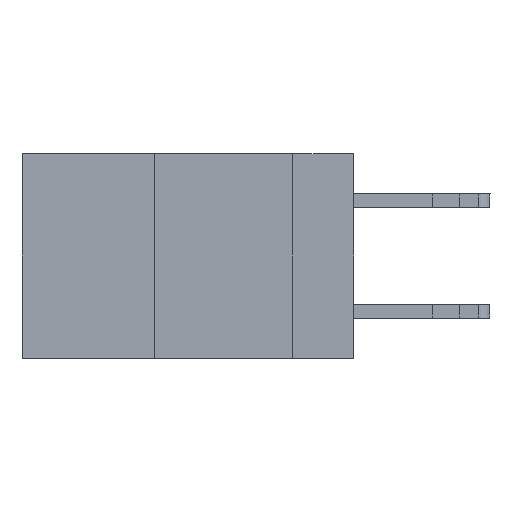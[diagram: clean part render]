
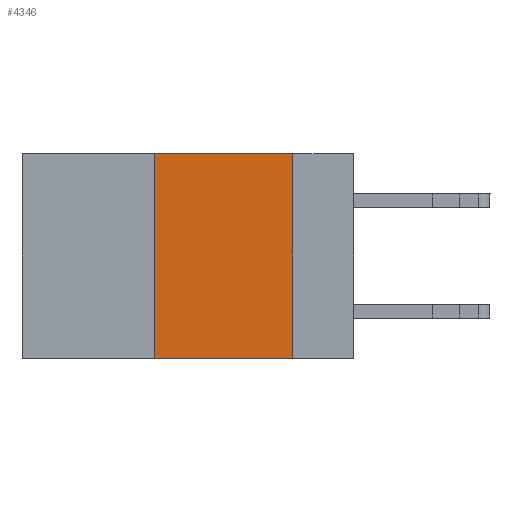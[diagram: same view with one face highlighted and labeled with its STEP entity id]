
A CAD part, left-side view. The second image highlights one B-rep face of the part: STEP entity #4346.
In plain terms, the highlighted planar face has unit normal (-1, 0, 0).
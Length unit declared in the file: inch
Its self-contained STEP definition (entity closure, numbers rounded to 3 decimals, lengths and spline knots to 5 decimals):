
#1619 = VECTOR ( 'NONE', #9592, 39.37008 ) ;
#1938 = VERTEX_POINT ( 'NONE', #3108 ) ;
#2101 = CARTESIAN_POINT ( 'NONE',  ( 0., 0.36, 0. ) ) ;
#2422 = EDGE_CURVE ( 'NONE', #11448, #7695, #15321, .T. ) ;
#2758 = CARTESIAN_POINT ( 'NONE',  ( 0., 0.11, -0.37 ) ) ;
#3108 = CARTESIAN_POINT ( 'NONE',  ( 0., 0.36, 0. ) ) ;
#4346 = ADVANCED_FACE ( 'NONE', ( #6828 ), #11741, .F. ) ;
#4435 = DIRECTION ( 'NONE',  ( 0., 0., -1. ) ) ;
#4913 = EDGE_CURVE ( 'NONE', #14951, #7695, #10792, .T. ) ;
#5261 = CARTESIAN_POINT ( 'NONE',  ( 0., 0.6, 0. ) ) ;
#5479 = EDGE_LOOP ( 'NONE', ( #7850, #7207, #13230, #13426 ) ) ;
#5728 = AXIS2_PLACEMENT_3D ( 'NONE', #7789, #10528, #4435 ) ;
#6042 = DIRECTION ( 'NONE',  ( 0., 0., 1. ) ) ;
#6828 = FACE_OUTER_BOUND ( 'NONE', #5479, .T. ) ;
#6985 = CARTESIAN_POINT ( 'NONE',  ( 0., 0.11, 0. ) ) ;
#7207 = ORIENTED_EDGE ( 'NONE', *, *, #12472, .F. ) ;
#7695 = VERTEX_POINT ( 'NONE', #2758 ) ;
#7789 = CARTESIAN_POINT ( 'NONE',  ( 0., 0.6, 0. ) ) ;
#7850 = ORIENTED_EDGE ( 'NONE', *, *, #4913, .F. ) ;
#8450 = VECTOR ( 'NONE', #6042, 39.37008 ) ;
#9592 = DIRECTION ( 'NONE',  ( 0., 0., -1. ) ) ;
#9771 = VECTOR ( 'NONE', #15555, 39.37008 ) ;
#10160 = DIRECTION ( 'NONE',  ( 0., -1., 0. ) ) ;
#10528 = DIRECTION ( 'NONE',  ( 1., 0., 0. ) ) ;
#10792 = LINE ( 'NONE', #14508, #1619 ) ;
#10986 = CARTESIAN_POINT ( 'NONE',  ( 0., 0.36, -0.37 ) ) ;
#11448 = VERTEX_POINT ( 'NONE', #10986 ) ;
#11741 = PLANE ( 'NONE',  #5728 ) ;
#12237 = VECTOR ( 'NONE', #10160, 39.37008 ) ;
#12472 = EDGE_CURVE ( 'NONE', #1938, #14951, #14918, .T. ) ;
#13230 = ORIENTED_EDGE ( 'NONE', *, *, #14507, .F. ) ;
#13426 = ORIENTED_EDGE ( 'NONE', *, *, #2422, .T. ) ;
#14261 = CARTESIAN_POINT ( 'NONE',  ( 0., 0.6, -0.37 ) ) ;
#14488 = LINE ( 'NONE', #2101, #8450 ) ;
#14507 = EDGE_CURVE ( 'NONE', #11448, #1938, #14488, .T. ) ;
#14508 = CARTESIAN_POINT ( 'NONE',  ( 0., 0.11, 0. ) ) ;
#14918 = LINE ( 'NONE', #5261, #12237 ) ;
#14951 = VERTEX_POINT ( 'NONE', #6985 ) ;
#15321 = LINE ( 'NONE', #14261, #9771 ) ;
#15555 = DIRECTION ( 'NONE',  ( 0., -1., 0. ) ) ;
